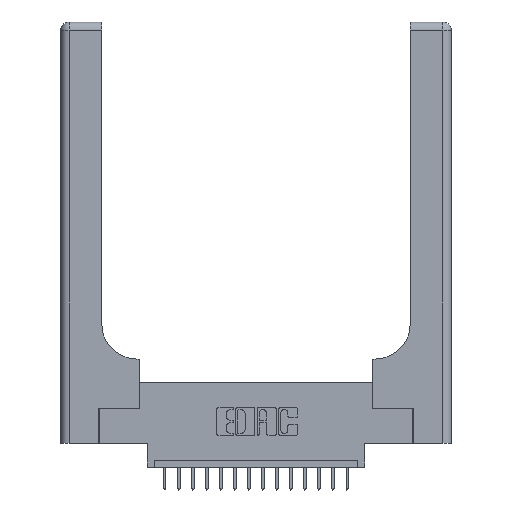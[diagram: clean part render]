
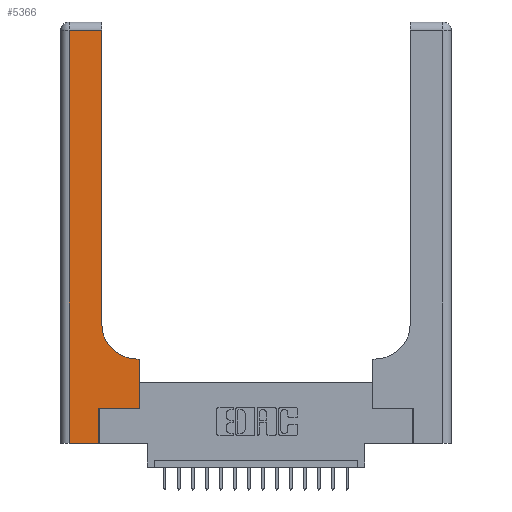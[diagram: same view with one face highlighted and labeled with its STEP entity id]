
A CAD part, top view. The second image highlights one B-rep face of the part: STEP entity #5366.
In plain terms, the highlighted planar face has unit normal (0, 0, 1).
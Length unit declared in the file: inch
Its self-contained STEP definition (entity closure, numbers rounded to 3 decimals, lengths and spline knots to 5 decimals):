
#817 = VECTOR ( 'NONE', #5511, 39.37008 ) ;
#839 = VERTEX_POINT ( 'NONE', #8215 ) ;
#1139 = CARTESIAN_POINT ( 'NONE',  ( 0.5585, 0.6, 0.37 ) ) ;
#1390 = CARTESIAN_POINT ( 'NONE',  ( 0.2915, 0.85, 0.37 ) ) ;
#1561 = VECTOR ( 'NONE', #2304, 39.37008 ) ;
#1709 = VERTEX_POINT ( 'NONE', #19092 ) ;
#1774 = CARTESIAN_POINT ( 'NONE',  ( 0.2915, 2.94, 0.37 ) ) ;
#1820 = CARTESIAN_POINT ( 'NONE',  ( 0., 0., 0.37 ) ) ;
#2238 = VECTOR ( 'NONE', #14886, 39.37008 ) ;
#2304 = DIRECTION ( 'NONE',  ( 0., -1., 0. ) ) ;
#2342 = DIRECTION ( 'NONE',  ( 1., 0., 0. ) ) ;
#2526 = DIRECTION ( 'NONE',  ( 0., 1., 0. ) ) ;
#2829 = VECTOR ( 'NONE', #2526, 39.37008 ) ;
#2971 = EDGE_CURVE ( 'NONE', #839, #1709, #13702, .T. ) ;
#3191 = EDGE_CURVE ( 'NONE', #1709, #13238, #7751, .T. ) ;
#3360 = DIRECTION ( 'NONE',  ( -1., 0., 0. ) ) ;
#3430 = CARTESIAN_POINT ( 'NONE',  ( 0., 2.94, 0.37 ) ) ;
#3818 = VECTOR ( 'NONE', #2342, 39.37008 ) ;
#3855 = EDGE_CURVE ( 'NONE', #15506, #16138, #13921, .T. ) ;
#3889 = CARTESIAN_POINT ( 'NONE',  ( 0.2915, 3., 0.37 ) ) ;
#4310 = EDGE_CURVE ( 'NONE', #13238, #14548, #8665, .T. ) ;
#5102 = CARTESIAN_POINT ( 'NONE',  ( 0., 3., 0.37 ) ) ;
#5366 = ADVANCED_FACE ( 'NONE', ( #11949 ), #8096, .F. ) ;
#5511 = DIRECTION ( 'NONE',  ( -1., 0., 0. ) ) ;
#5806 = ORIENTED_EDGE ( 'NONE', *, *, #5902, .T. ) ;
#5840 = DIRECTION ( 'NONE',  ( 1., 0., 0. ) ) ;
#5902 = EDGE_CURVE ( 'NONE', #14548, #16363, #15948, .T. ) ;
#6224 = ORIENTED_EDGE ( 'NONE', *, *, #2971, .T. ) ;
#6391 = DIRECTION ( 'NONE',  ( 1., 0., 0. ) ) ;
#6539 = ORIENTED_EDGE ( 'NONE', *, *, #3191, .T. ) ;
#7365 = VECTOR ( 'NONE', #3360, 39.37008 ) ;
#7406 = EDGE_LOOP ( 'NONE', ( #15273, #11321, #6224, #6539, #15383, #5806, #7642, #19189, #10846 ) ) ;
#7642 = ORIENTED_EDGE ( 'NONE', *, *, #12604, .T. ) ;
#7751 = LINE ( 'NONE', #1820, #13489 ) ;
#8046 = EDGE_CURVE ( 'NONE', #18812, #11411, #18717, .T. ) ;
#8096 = PLANE ( 'NONE',  #8369 ) ;
#8215 = CARTESIAN_POINT ( 'NONE',  ( 0.06, 2.94, 0.37 ) ) ;
#8369 = AXIS2_PLACEMENT_3D ( 'NONE', #5102, #15721, #14282 ) ;
#8665 = LINE ( 'NONE', #17544, #2238 ) ;
#9859 = CARTESIAN_POINT ( 'NONE',  ( 0.269, 0., 0.37 ) ) ;
#10235 = CARTESIAN_POINT ( 'NONE',  ( 0.5585, 0.25, 0.37 ) ) ;
#10846 = ORIENTED_EDGE ( 'NONE', *, *, #15553, .T. ) ;
#11321 = ORIENTED_EDGE ( 'NONE', *, *, #19007, .T. ) ;
#11411 = VERTEX_POINT ( 'NONE', #1774 ) ;
#11416 = LINE ( 'NONE', #3430, #7365 ) ;
#11949 = FACE_OUTER_BOUND ( 'NONE', #7406, .T. ) ;
#12321 = VECTOR ( 'NONE', #13022, 39.37008 ) ;
#12604 = EDGE_CURVE ( 'NONE', #16363, #15506, #15897, .T. ) ;
#13022 = DIRECTION ( 'NONE',  ( 0., 1., 0. ) ) ;
#13238 = VERTEX_POINT ( 'NONE', #9859 ) ;
#13489 = VECTOR ( 'NONE', #6391, 39.37008 ) ;
#13702 = LINE ( 'NONE', #14330, #1561 ) ;
#13921 = LINE ( 'NONE', #19145, #817 ) ;
#14071 = CARTESIAN_POINT ( 'NONE',  ( 0.269, 0.25, 0.37 ) ) ;
#14282 = DIRECTION ( 'NONE',  ( -1., 0., 0. ) ) ;
#14330 = CARTESIAN_POINT ( 'NONE',  ( 0.06, 3., 0.37 ) ) ;
#14447 = AXIS2_PLACEMENT_3D ( 'NONE', #18072, #19492, #5840 ) ;
#14548 = VERTEX_POINT ( 'NONE', #14071 ) ;
#14886 = DIRECTION ( 'NONE',  ( 0., 1., 0. ) ) ;
#14919 = CARTESIAN_POINT ( 'NONE',  ( 0.5415, 0.6, 0.37 ) ) ;
#15273 = ORIENTED_EDGE ( 'NONE', *, *, #8046, .T. ) ;
#15383 = ORIENTED_EDGE ( 'NONE', *, *, #4310, .T. ) ;
#15506 = VERTEX_POINT ( 'NONE', #1139 ) ;
#15553 = EDGE_CURVE ( 'NONE', #16138, #18812, #16782, .T. ) ;
#15721 = DIRECTION ( 'NONE',  ( 0., 0., -1. ) ) ;
#15897 = LINE ( 'NONE', #10235, #2829 ) ;
#15948 = LINE ( 'NONE', #19012, #3818 ) ;
#16138 = VERTEX_POINT ( 'NONE', #14919 ) ;
#16363 = VERTEX_POINT ( 'NONE', #17695 ) ;
#16782 = CIRCLE ( 'NONE', #14447, 0.25 ) ;
#17544 = CARTESIAN_POINT ( 'NONE',  ( 0.269, 0., 0.37 ) ) ;
#17695 = CARTESIAN_POINT ( 'NONE',  ( 0.5585, 0.25, 0.37 ) ) ;
#18072 = CARTESIAN_POINT ( 'NONE',  ( 0.5415, 0.85, 0.37 ) ) ;
#18717 = LINE ( 'NONE', #3889, #12321 ) ;
#18812 = VERTEX_POINT ( 'NONE', #1390 ) ;
#19007 = EDGE_CURVE ( 'NONE', #11411, #839, #11416, .T. ) ;
#19012 = CARTESIAN_POINT ( 'NONE',  ( 0.269, 0.25, 0.37 ) ) ;
#19092 = CARTESIAN_POINT ( 'NONE',  ( 0.06, 0., 0.37 ) ) ;
#19145 = CARTESIAN_POINT ( 'NONE',  ( 0.2915, 0.6, 0.37 ) ) ;
#19189 = ORIENTED_EDGE ( 'NONE', *, *, #3855, .T. ) ;
#19492 = DIRECTION ( 'NONE',  ( 0., 0., -1. ) ) ;
